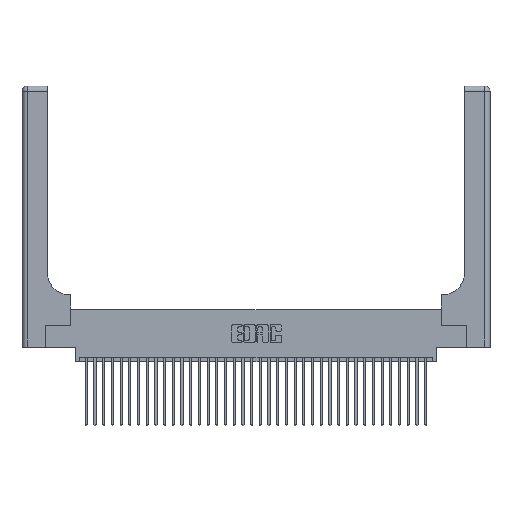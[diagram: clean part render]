
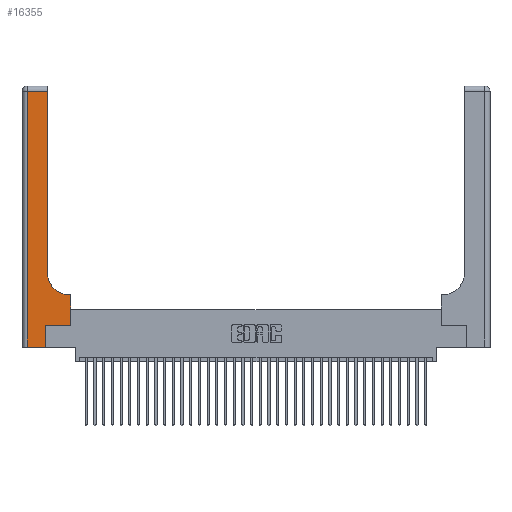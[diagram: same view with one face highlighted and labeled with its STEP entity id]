
A CAD part, top view. The second image highlights one B-rep face of the part: STEP entity #16355.
In plain terms, the highlighted planar face has unit normal (0, 0, 1).
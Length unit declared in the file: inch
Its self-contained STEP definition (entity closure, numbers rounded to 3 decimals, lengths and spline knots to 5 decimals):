
#1033 = ORIENTED_EDGE ( 'NONE', *, *, #16532, .T. ) ;
#1163 = LINE ( 'NONE', #7547, #28581 ) ;
#1717 = EDGE_CURVE ( 'NONE', #34956, #24501, #21404, .T. ) ;
#1882 = EDGE_CURVE ( 'NONE', #13621, #6240, #15611, .T. ) ;
#2037 = VECTOR ( 'NONE', #13395, 39.37008 ) ;
#3372 = LINE ( 'NONE', #23374, #4762 ) ;
#3523 = DIRECTION ( 'NONE',  ( 0., 1., 0. ) ) ;
#4480 = DIRECTION ( 'NONE',  ( -1., 0., 0. ) ) ;
#4586 = EDGE_LOOP ( 'NONE', ( #1033, #29726, #16286, #18596, #8559, #10377, #12072, #29957, #20366 ) ) ;
#4629 = DIRECTION ( 'NONE',  ( 1., 0., 0. ) ) ;
#4640 = EDGE_CURVE ( 'NONE', #15833, #13621, #35478, .T. ) ;
#4762 = VECTOR ( 'NONE', #3523, 39.37008 ) ;
#4940 = AXIS2_PLACEMENT_3D ( 'NONE', #21242, #35130, #16896 ) ;
#5045 = CARTESIAN_POINT ( 'NONE',  ( 0.5585, 0.25, 0.37 ) ) ;
#5501 = LINE ( 'NONE', #30657, #9901 ) ;
#6091 = VERTEX_POINT ( 'NONE', #29712 ) ;
#6240 = VERTEX_POINT ( 'NONE', #32734 ) ;
#7333 = CARTESIAN_POINT ( 'NONE',  ( 0.5585, 0.25, 0.37 ) ) ;
#7510 = VERTEX_POINT ( 'NONE', #30052 ) ;
#7547 = CARTESIAN_POINT ( 'NONE',  ( 0.269, 0., 0.37 ) ) ;
#8559 = ORIENTED_EDGE ( 'NONE', *, *, #11662, .T. ) ;
#9148 = VECTOR ( 'NONE', #18104, 39.37008 ) ;
#9713 = CARTESIAN_POINT ( 'NONE',  ( 0.269, 0.25, 0.37 ) ) ;
#9901 = VECTOR ( 'NONE', #25087, 39.37008 ) ;
#10068 = CARTESIAN_POINT ( 'NONE',  ( 0.269, 0., 0.37 ) ) ;
#10142 = EDGE_CURVE ( 'NONE', #6240, #35186, #25155, .T. ) ;
#10151 = CIRCLE ( 'NONE', #33364, 0.25 ) ;
#10377 = ORIENTED_EDGE ( 'NONE', *, *, #4640, .T. ) ;
#11662 = EDGE_CURVE ( 'NONE', #24501, #15833, #1163, .T. ) ;
#12072 = ORIENTED_EDGE ( 'NONE', *, *, #1882, .T. ) ;
#12805 = DIRECTION ( 'NONE',  ( 1., 0., 0. ) ) ;
#13190 = CARTESIAN_POINT ( 'NONE',  ( 0.2915, 0.6, 0.37 ) ) ;
#13395 = DIRECTION ( 'NONE',  ( 1., 0., 0. ) ) ;
#13621 = VERTEX_POINT ( 'NONE', #7333 ) ;
#13691 = PLANE ( 'NONE',  #4940 ) ;
#14493 = CARTESIAN_POINT ( 'NONE',  ( 0.06, 0., 0.37 ) ) ;
#15412 = FACE_OUTER_BOUND ( 'NONE', #4586, .T. ) ;
#15611 = LINE ( 'NONE', #5045, #19693 ) ;
#15833 = VERTEX_POINT ( 'NONE', #9713 ) ;
#16286 = ORIENTED_EDGE ( 'NONE', *, *, #36237, .T. ) ;
#16355 = ADVANCED_FACE ( 'NONE', ( #15412 ), #13691, .F. ) ;
#16532 = EDGE_CURVE ( 'NONE', #29091, #6091, #3372, .T. ) ;
#16896 = DIRECTION ( 'NONE',  ( -1., 0., 0. ) ) ;
#18104 = DIRECTION ( 'NONE',  ( 0., -1., 0. ) ) ;
#18596 = ORIENTED_EDGE ( 'NONE', *, *, #1717, .T. ) ;
#18876 = CARTESIAN_POINT ( 'NONE',  ( 0.269, 0.25, 0.37 ) ) ;
#19693 = VECTOR ( 'NONE', #33737, 39.37008 ) ;
#20366 = ORIENTED_EDGE ( 'NONE', *, *, #25101, .T. ) ;
#21242 = CARTESIAN_POINT ( 'NONE',  ( 0., 3., 0.37 ) ) ;
#21404 = LINE ( 'NONE', #29560, #31714 ) ;
#22712 = EDGE_CURVE ( 'NONE', #6091, #7510, #5501, .T. ) ;
#23374 = CARTESIAN_POINT ( 'NONE',  ( 0.2915, 3., 0.37 ) ) ;
#24167 = VECTOR ( 'NONE', #4480, 39.37008 ) ;
#24454 = CARTESIAN_POINT ( 'NONE',  ( 0.5415, 0.85, 0.37 ) ) ;
#24501 = VERTEX_POINT ( 'NONE', #10068 ) ;
#25087 = DIRECTION ( 'NONE',  ( -1., 0., 0. ) ) ;
#25101 = EDGE_CURVE ( 'NONE', #35186, #29091, #10151, .T. ) ;
#25155 = LINE ( 'NONE', #13190, #24167 ) ;
#26520 = LINE ( 'NONE', #32315, #9148 ) ;
#27511 = DIRECTION ( 'NONE',  ( 0., 1., 0. ) ) ;
#28581 = VECTOR ( 'NONE', #27511, 39.37008 ) ;
#29091 = VERTEX_POINT ( 'NONE', #29404 ) ;
#29404 = CARTESIAN_POINT ( 'NONE',  ( 0.2915, 0.85, 0.37 ) ) ;
#29560 = CARTESIAN_POINT ( 'NONE',  ( 0., 0., 0.37 ) ) ;
#29712 = CARTESIAN_POINT ( 'NONE',  ( 0.2915, 2.94, 0.37 ) ) ;
#29726 = ORIENTED_EDGE ( 'NONE', *, *, #22712, .T. ) ;
#29957 = ORIENTED_EDGE ( 'NONE', *, *, #10142, .T. ) ;
#30052 = CARTESIAN_POINT ( 'NONE',  ( 0.06, 2.94, 0.37 ) ) ;
#30657 = CARTESIAN_POINT ( 'NONE',  ( 0., 2.94, 0.37 ) ) ;
#31714 = VECTOR ( 'NONE', #4629, 39.37008 ) ;
#32315 = CARTESIAN_POINT ( 'NONE',  ( 0.06, 3., 0.37 ) ) ;
#32734 = CARTESIAN_POINT ( 'NONE',  ( 0.5585, 0.6, 0.37 ) ) ;
#33323 = DIRECTION ( 'NONE',  ( 0., 0., -1. ) ) ;
#33364 = AXIS2_PLACEMENT_3D ( 'NONE', #24454, #33323, #12805 ) ;
#33737 = DIRECTION ( 'NONE',  ( 0., 1., 0. ) ) ;
#34956 = VERTEX_POINT ( 'NONE', #14493 ) ;
#35130 = DIRECTION ( 'NONE',  ( 0., 0., -1. ) ) ;
#35186 = VERTEX_POINT ( 'NONE', #36211 ) ;
#35478 = LINE ( 'NONE', #18876, #2037 ) ;
#36211 = CARTESIAN_POINT ( 'NONE',  ( 0.5415, 0.6, 0.37 ) ) ;
#36237 = EDGE_CURVE ( 'NONE', #7510, #34956, #26520, .T. ) ;
